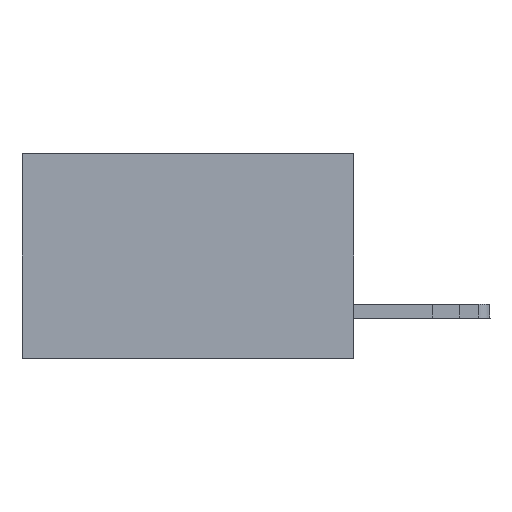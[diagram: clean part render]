
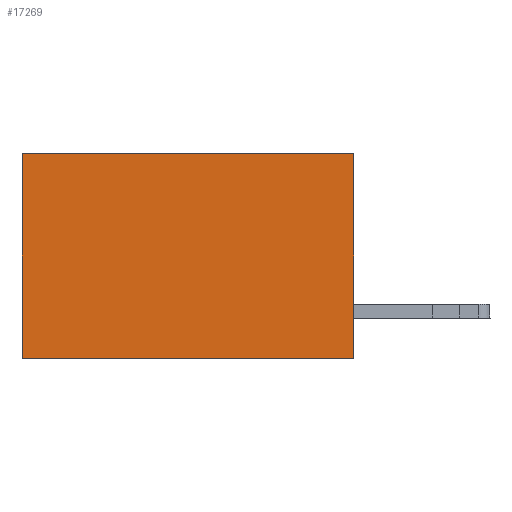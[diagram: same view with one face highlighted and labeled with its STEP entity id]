
A CAD part, left-side view. The second image highlights one B-rep face of the part: STEP entity #17269.
In plain terms, the highlighted planar face has unit normal (-1, 0, 0).
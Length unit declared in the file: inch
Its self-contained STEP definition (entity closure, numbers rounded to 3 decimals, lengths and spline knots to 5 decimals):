
#364 = VERTEX_POINT ( 'NONE', #16744 ) ;
#373 = CARTESIAN_POINT ( 'NONE',  ( 0.2875, 0.6, 0. ) ) ;
#558 = EDGE_CURVE ( 'NONE', #872, #20515, #18885, .T. ) ;
#714 = CARTESIAN_POINT ( 'NONE',  ( 0.2875, 0., 0. ) ) ;
#872 = VERTEX_POINT ( 'NONE', #24347 ) ;
#2091 = LINE ( 'NONE', #20927, #21606 ) ;
#2123 = FACE_OUTER_BOUND ( 'NONE', #10990, .T. ) ;
#2280 = CARTESIAN_POINT ( 'NONE',  ( 0.2875, 0.6, -0.37 ) ) ;
#3610 = VECTOR ( 'NONE', #25367, 39.37008 ) ;
#3684 = DIRECTION ( 'NONE',  ( 1., 0., 0. ) ) ;
#5291 = EDGE_CURVE ( 'NONE', #364, #8470, #18212, .T. ) ;
#7056 = AXIS2_PLACEMENT_3D ( 'NONE', #12253, #3684, #18249 ) ;
#8470 = VERTEX_POINT ( 'NONE', #2280 ) ;
#10990 = EDGE_LOOP ( 'NONE', ( #16207, #16000, #20958, #17033 ) ) ;
#11010 = VECTOR ( 'NONE', #23929, 39.37008 ) ;
#12253 = CARTESIAN_POINT ( 'NONE',  ( 0.2875, 0., 0. ) ) ;
#13278 = CARTESIAN_POINT ( 'NONE',  ( 0.2875, 0., -0.37 ) ) ;
#15254 = EDGE_CURVE ( 'NONE', #872, #364, #20414, .T. ) ;
#16000 = ORIENTED_EDGE ( 'NONE', *, *, #5291, .F. ) ;
#16134 = PLANE ( 'NONE',  #7056 ) ;
#16207 = ORIENTED_EDGE ( 'NONE', *, *, #17367, .T. ) ;
#16744 = CARTESIAN_POINT ( 'NONE',  ( 0.2875, 0., -0.37 ) ) ;
#17033 = ORIENTED_EDGE ( 'NONE', *, *, #558, .T. ) ;
#17112 = DIRECTION ( 'NONE',  ( 0., 0., -1. ) ) ;
#17146 = CARTESIAN_POINT ( 'NONE',  ( 0.2875, 0., 0. ) ) ;
#17269 = ADVANCED_FACE ( 'NONE', ( #2123 ), #16134, .F. ) ;
#17367 = EDGE_CURVE ( 'NONE', #20515, #8470, #2091, .T. ) ;
#18212 = LINE ( 'NONE', #13278, #19802 ) ;
#18249 = DIRECTION ( 'NONE',  ( 0., 0., -1. ) ) ;
#18885 = LINE ( 'NONE', #714, #3610 ) ;
#19802 = VECTOR ( 'NONE', #25457, 39.37008 ) ;
#20414 = LINE ( 'NONE', #17146, #11010 ) ;
#20515 = VERTEX_POINT ( 'NONE', #373 ) ;
#20927 = CARTESIAN_POINT ( 'NONE',  ( 0.2875, 0.6, 0. ) ) ;
#20958 = ORIENTED_EDGE ( 'NONE', *, *, #15254, .F. ) ;
#21606 = VECTOR ( 'NONE', #17112, 39.37008 ) ;
#23929 = DIRECTION ( 'NONE',  ( 0., 0., -1. ) ) ;
#24347 = CARTESIAN_POINT ( 'NONE',  ( 0.2875, 0., 0. ) ) ;
#25367 = DIRECTION ( 'NONE',  ( 0., 1., 0. ) ) ;
#25457 = DIRECTION ( 'NONE',  ( 0., 1., 0. ) ) ;
